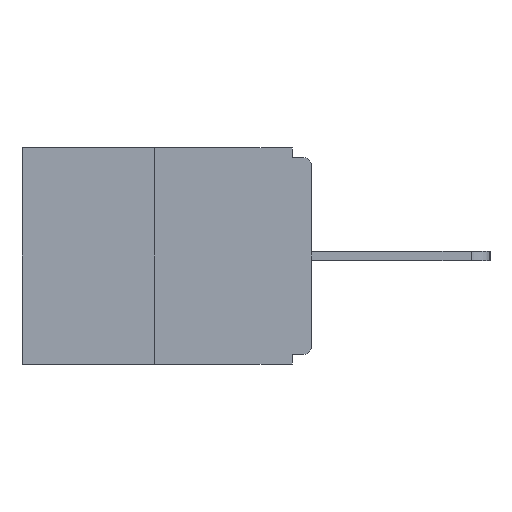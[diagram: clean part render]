
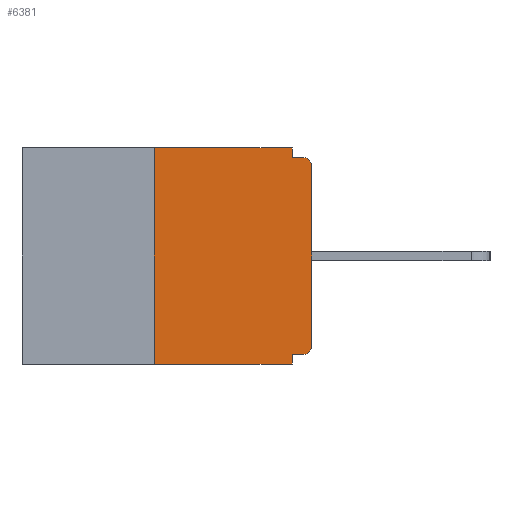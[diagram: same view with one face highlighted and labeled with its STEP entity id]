
A CAD part, left-side view. The second image highlights one B-rep face of the part: STEP entity #6381.
In plain terms, the highlighted planar face has unit normal (-1, 0, 0).
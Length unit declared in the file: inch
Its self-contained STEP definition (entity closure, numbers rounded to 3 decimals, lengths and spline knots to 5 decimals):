
#148 = EDGE_CURVE ( 'NONE', #2757, #9832, #13012, .T. ) ;
#154 = PLANE ( 'NONE',  #9979 ) ;
#172 = VECTOR ( 'NONE', #9822, 39.37008 ) ;
#726 = DIRECTION ( 'NONE',  ( 0., -1., 0. ) ) ;
#1197 = CIRCLE ( 'NONE', #1455, 0.015 ) ;
#1236 = ORIENTED_EDGE ( 'NONE', *, *, #13882, .T. ) ;
#1309 = CARTESIAN_POINT ( 'NONE',  ( 0., 0.46, 0. ) ) ;
#1356 = CARTESIAN_POINT ( 'NONE',  ( 0., 0.031, -0.328 ) ) ;
#1455 = AXIS2_PLACEMENT_3D ( 'NONE', #11897, #4641, #13111 ) ;
#2315 = VERTEX_POINT ( 'NONE', #9501 ) ;
#2442 = LINE ( 'NONE', #8800, #8506 ) ;
#2448 = ORIENTED_EDGE ( 'NONE', *, *, #5149, .T. ) ;
#2757 = VERTEX_POINT ( 'NONE', #12758 ) ;
#3192 = DIRECTION ( 'NONE',  ( 0., 1., 0. ) ) ;
#3431 = ORIENTED_EDGE ( 'NONE', *, *, #4823, .F. ) ;
#3456 = LINE ( 'NONE', #10947, #9555 ) ;
#3626 = CARTESIAN_POINT ( 'NONE',  ( 0., 0.031, -0.015 ) ) ;
#3685 = EDGE_CURVE ( 'NONE', #14428, #5951, #5518, .T. ) ;
#3741 = DIRECTION ( 'NONE',  ( 0., 0., -1. ) ) ;
#3744 = CARTESIAN_POINT ( 'NONE',  ( 0., 0.46, -0.343 ) ) ;
#3761 = FACE_OUTER_BOUND ( 'NONE', #6899, .T. ) ;
#4371 = CARTESIAN_POINT ( 'NONE',  ( 0., 0.031, -0.343 ) ) ;
#4512 = EDGE_CURVE ( 'NONE', #8113, #14976, #3456, .T. ) ;
#4641 = DIRECTION ( 'NONE',  ( -1., 0., 0. ) ) ;
#4646 = VECTOR ( 'NONE', #9786, 39.37008 ) ;
#4808 = VECTOR ( 'NONE', #5604, 39.37008 ) ;
#4823 = EDGE_CURVE ( 'NONE', #14976, #10795, #8206, .T. ) ;
#5149 = EDGE_CURVE ( 'NONE', #14428, #9329, #1197, .T. ) ;
#5186 = CARTESIAN_POINT ( 'NONE',  ( 0., 0.015, -0.03 ) ) ;
#5518 = LINE ( 'NONE', #12873, #14820 ) ;
#5574 = LINE ( 'NONE', #4371, #4808 ) ;
#5604 = DIRECTION ( 'NONE',  ( 0., 0., -1. ) ) ;
#5648 = CARTESIAN_POINT ( 'NONE',  ( 0., 0., 0. ) ) ;
#5951 = VERTEX_POINT ( 'NONE', #1356 ) ;
#6213 = CARTESIAN_POINT ( 'NONE',  ( 0., 0., -0.03 ) ) ;
#6381 = ADVANCED_FACE ( 'NONE', ( #3761 ), #154, .F. ) ;
#6417 = DIRECTION ( 'NONE',  ( 0., 0., -1. ) ) ;
#6899 = EDGE_LOOP ( 'NONE', ( #13073, #13703, #12847, #11934, #8592, #2448, #1236, #9973, #3431, #11309 ) ) ;
#6995 = EDGE_CURVE ( 'NONE', #2757, #2315, #2442, .T. ) ;
#7887 = LINE ( 'NONE', #1309, #4646 ) ;
#7939 = CARTESIAN_POINT ( 'NONE',  ( 0., 0., -0.015 ) ) ;
#8113 = VERTEX_POINT ( 'NONE', #13382 ) ;
#8206 = LINE ( 'NONE', #7939, #11417 ) ;
#8506 = VECTOR ( 'NONE', #13587, 39.37008 ) ;
#8592 = ORIENTED_EDGE ( 'NONE', *, *, #3685, .F. ) ;
#8744 = EDGE_CURVE ( 'NONE', #2315, #8113, #7887, .T. ) ;
#8800 = CARTESIAN_POINT ( 'NONE',  ( 0., 0.25, 0. ) ) ;
#9329 = VERTEX_POINT ( 'NONE', #9828 ) ;
#9501 = CARTESIAN_POINT ( 'NONE',  ( 0., 0.25, 0. ) ) ;
#9555 = VECTOR ( 'NONE', #12178, 39.37008 ) ;
#9786 = DIRECTION ( 'NONE',  ( 0., -1., 0. ) ) ;
#9822 = DIRECTION ( 'NONE',  ( 0., -1., 0. ) ) ;
#9828 = CARTESIAN_POINT ( 'NONE',  ( 0., 0., -0.313 ) ) ;
#9832 = VERTEX_POINT ( 'NONE', #10849 ) ;
#9973 = ORIENTED_EDGE ( 'NONE', *, *, #13076, .T. ) ;
#9979 = AXIS2_PLACEMENT_3D ( 'NONE', #12124, #11018, #3741 ) ;
#10338 = AXIS2_PLACEMENT_3D ( 'NONE', #5186, #13658, #6417 ) ;
#10795 = VERTEX_POINT ( 'NONE', #14285 ) ;
#10802 = CIRCLE ( 'NONE', #10338, 0.015 ) ;
#10849 = CARTESIAN_POINT ( 'NONE',  ( 0., 0.031, -0.343 ) ) ;
#10865 = VECTOR ( 'NONE', #15337, 39.37008 ) ;
#10947 = CARTESIAN_POINT ( 'NONE',  ( 0., 0.031, 0. ) ) ;
#11018 = DIRECTION ( 'NONE',  ( 1., 0., 0. ) ) ;
#11250 = LINE ( 'NONE', #5648, #10865 ) ;
#11309 = ORIENTED_EDGE ( 'NONE', *, *, #4512, .F. ) ;
#11417 = VECTOR ( 'NONE', #726, 39.37008 ) ;
#11897 = CARTESIAN_POINT ( 'NONE',  ( 0., 0.015, -0.313 ) ) ;
#11934 = ORIENTED_EDGE ( 'NONE', *, *, #13845, .F. ) ;
#12124 = CARTESIAN_POINT ( 'NONE',  ( 0., 0.46, 0. ) ) ;
#12178 = DIRECTION ( 'NONE',  ( 0., 0., -1. ) ) ;
#12758 = CARTESIAN_POINT ( 'NONE',  ( 0., 0.25, -0.343 ) ) ;
#12847 = ORIENTED_EDGE ( 'NONE', *, *, #148, .T. ) ;
#12873 = CARTESIAN_POINT ( 'NONE',  ( 0., 0., -0.328 ) ) ;
#13012 = LINE ( 'NONE', #3744, #172 ) ;
#13073 = ORIENTED_EDGE ( 'NONE', *, *, #8744, .F. ) ;
#13076 = EDGE_CURVE ( 'NONE', #14770, #10795, #10802, .T. ) ;
#13111 = DIRECTION ( 'NONE',  ( 0., 0., -1. ) ) ;
#13382 = CARTESIAN_POINT ( 'NONE',  ( 0., 0.031, 0. ) ) ;
#13587 = DIRECTION ( 'NONE',  ( 0., 0., 1. ) ) ;
#13658 = DIRECTION ( 'NONE',  ( -1., 0., 0. ) ) ;
#13703 = ORIENTED_EDGE ( 'NONE', *, *, #6995, .F. ) ;
#13845 = EDGE_CURVE ( 'NONE', #5951, #9832, #5574, .T. ) ;
#13882 = EDGE_CURVE ( 'NONE', #9329, #14770, #11250, .T. ) ;
#14044 = CARTESIAN_POINT ( 'NONE',  ( 0., 0.015, -0.328 ) ) ;
#14285 = CARTESIAN_POINT ( 'NONE',  ( 0., 0.015, -0.015 ) ) ;
#14428 = VERTEX_POINT ( 'NONE', #14044 ) ;
#14770 = VERTEX_POINT ( 'NONE', #6213 ) ;
#14820 = VECTOR ( 'NONE', #3192, 39.37008 ) ;
#14976 = VERTEX_POINT ( 'NONE', #3626 ) ;
#15337 = DIRECTION ( 'NONE',  ( 0., 0., 1. ) ) ;
